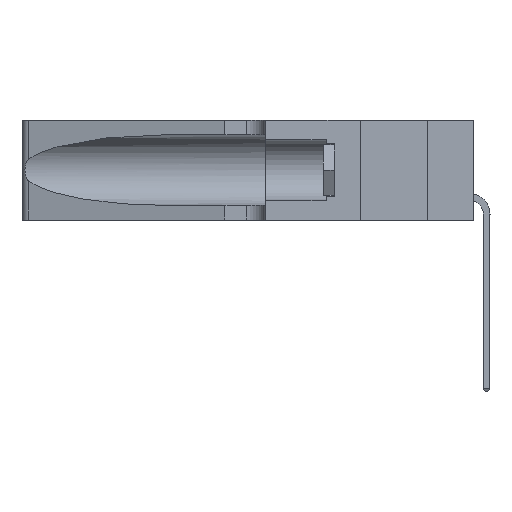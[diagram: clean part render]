
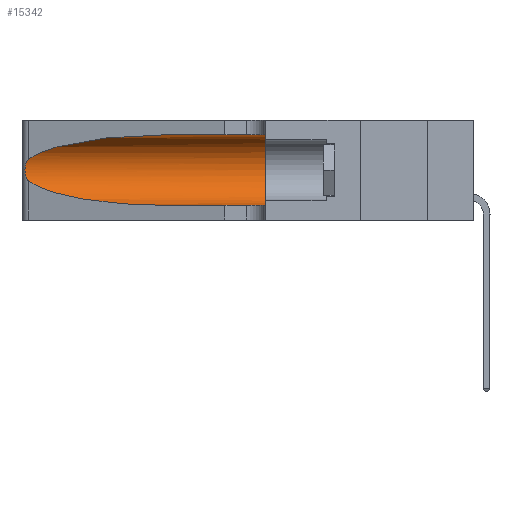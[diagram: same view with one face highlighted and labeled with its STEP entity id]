
A CAD part, left-side view. The second image highlights one B-rep face of the part: STEP entity #15342.
In plain terms, the highlighted cylindrical face has radius 3.308 mm (diameter 6.617 mm), a partial arc.
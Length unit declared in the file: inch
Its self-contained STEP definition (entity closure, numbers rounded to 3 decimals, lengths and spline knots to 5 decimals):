
#10 = B_SPLINE_CURVE_WITH_KNOTS ( 'NONE', 3,
 ( #20231, #10800, #4668, #15788, #2941, #12462, #14384, #12871, #17435, #11341, #9580, #4878, #15926, #14451 ),
 .UNSPECIFIED., .F., .F.,
 ( 4, 2, 2, 2, 2, 2, 4 ),
 ( 0., 0.00027, 0.00053, 0.00107, 0.0016, 0.00187, 0.00214 ),
 .UNSPECIFIED. ) ;
#601 = ORIENTED_EDGE ( 'NONE', *, *, #5058, .T. ) ;
#1097 = AXIS2_PLACEMENT_3D ( 'NONE', #1220, #7774, #7566 ) ;
#1220 = CARTESIAN_POINT ( 'NONE',  ( 0.1305, 0.35, 0.185 ) ) ;
#1369 = VERTEX_POINT ( 'NONE', #12164 ) ;
#1884 = CARTESIAN_POINT ( 'NONE',  ( 0.18966, 0.96281, 0.31525 ) ) ;
#2132 = DIRECTION ( 'NONE',  ( 0., 0., -1. ) ) ;
#2319 = CARTESIAN_POINT ( 'NONE',  ( 0.25487, 1.22718, 0.22369 ) ) ;
#2742 = CARTESIAN_POINT ( 'NONE',  ( 0.1305, 1.61858, 0.31525 ) ) ;
#2941 = CARTESIAN_POINT ( 'NONE',  ( 0.25854, 1.2359, 0.20912 ) ) ;
#3533 = VERTEX_POINT ( 'NONE', #2319 ) ;
#4243 = EDGE_CURVE ( 'NONE', #11460, #1369, #17446, .T. ) ;
#4668 = CARTESIAN_POINT ( 'NONE',  ( 0.25639, 1.23184, 0.21858 ) ) ;
#4878 = CARTESIAN_POINT ( 'NONE',  ( 0.25639, 1.23186, 0.15144 ) ) ;
#5058 = EDGE_CURVE ( 'NONE', #3533, #11460, #10, .T. ) ;
#5115 = CARTESIAN_POINT ( 'NONE',  ( 0.1305, 0.35, 0.31525 ) ) ;
#5627 = VERTEX_POINT ( 'NONE', #8941 ) ;
#6149 = EDGE_CURVE ( 'NONE', #8811, #18917, #12539, .T. ) ;
#6348 = DIRECTION ( 'NONE',  ( 0., -1., 0. ) ) ;
#6776 = ORIENTED_EDGE ( 'NONE', *, *, #20018, .T. ) ;
#6941 = CARTESIAN_POINT ( 'NONE',  ( 0.18966, 0.96281, 0.05475 ) ) ;
#7340 = EDGE_CURVE ( 'NONE', #1369, #5627, #11021, .T. ) ;
#7566 = DIRECTION ( 'NONE',  ( 0., 0., 1. ) ) ;
#7774 = DIRECTION ( 'NONE',  ( 0., 1., 0. ) ) ;
#7825 = EDGE_CURVE ( 'NONE', #18917, #5627, #13225, .T. ) ;
#8082 =( BOUNDED_CURVE ( )  B_SPLINE_CURVE ( 3, ( #8178, #1884, #8108, #9747 ),
 .UNSPECIFIED., .F., .F. ) 
 B_SPLINE_CURVE_WITH_KNOTS ( ( 4, 4 ),
 ( 1.5708, 2.84003 ),
 .UNSPECIFIED. ) 
 CURVE ( )  GEOMETRIC_REPRESENTATION_ITEM ( )  RATIONAL_B_SPLINE_CURVE ( ( 1., 0.87, 0.87, 1. ) ) 
 REPRESENTATION_ITEM ( '' )  );
#8108 = CARTESIAN_POINT ( 'NONE',  ( 0.2373, 1.15595, 0.28018 ) ) ;
#8178 = CARTESIAN_POINT ( 'NONE',  ( 0.1305, 0.72297, 0.31525 ) ) ;
#8194 = CARTESIAN_POINT ( 'NONE',  ( 0.1305, 0.72297, 0.31525 ) ) ;
#8485 = ORIENTED_EDGE ( 'NONE', *, *, #7825, .F. ) ;
#8613 = CARTESIAN_POINT ( 'NONE',  ( 0.1305, 1.61858, 0.185 ) ) ;
#8811 = VERTEX_POINT ( 'NONE', #8194 ) ;
#8941 = CARTESIAN_POINT ( 'NONE',  ( 0.1305, 0.35, 0.05475 ) ) ;
#9384 = CARTESIAN_POINT ( 'NONE',  ( 0.2373, 1.15595, 0.08982 ) ) ;
#9580 = CARTESIAN_POINT ( 'NONE',  ( 0.25789, 1.23486, 0.15765 ) ) ;
#9747 = CARTESIAN_POINT ( 'NONE',  ( 0.25487, 1.22718, 0.22369 ) ) ;
#10800 = CARTESIAN_POINT ( 'NONE',  ( 0.25555, 1.22994, 0.2215 ) ) ;
#11021 = LINE ( 'NONE', #15819, #19888 ) ;
#11341 = CARTESIAN_POINT ( 'NONE',  ( 0.25856, 1.23593, 0.16098 ) ) ;
#11460 = VERTEX_POINT ( 'NONE', #17697 ) ;
#11747 = DIRECTION ( 'NONE',  ( 0., -1., 0. ) ) ;
#11995 = ORIENTED_EDGE ( 'NONE', *, *, #4243, .T. ) ;
#12164 = CARTESIAN_POINT ( 'NONE',  ( 0.1305, 0.72297, 0.05475 ) ) ;
#12462 = CARTESIAN_POINT ( 'NONE',  ( 0.26018, 1.23835, 0.19895 ) ) ;
#12469 = CARTESIAN_POINT ( 'NONE',  ( 0.25487, 1.22718, 0.14631 ) ) ;
#12539 = LINE ( 'NONE', #2742, #17978 ) ;
#12781 = EDGE_LOOP ( 'NONE', ( #6776, #601, #11995, #20378, #8485, #14394 ) ) ;
#12871 = CARTESIAN_POINT ( 'NONE',  ( 0.26075, 1.23896, 0.178 ) ) ;
#12925 = CYLINDRICAL_SURFACE ( 'NONE', #15602, 0.13025 ) ;
#13176 = FACE_OUTER_BOUND ( 'NONE', #12781, .T. ) ;
#13225 = CIRCLE ( 'NONE', #1097, 0.13025 ) ;
#14384 = CARTESIAN_POINT ( 'NONE',  ( 0.26075, 1.23896, 0.19203 ) ) ;
#14394 = ORIENTED_EDGE ( 'NONE', *, *, #6149, .F. ) ;
#14451 = CARTESIAN_POINT ( 'NONE',  ( 0.25487, 1.22718, 0.14631 ) ) ;
#15342 = ADVANCED_FACE ( 'NONE', ( #13176 ), #12925, .F. ) ;
#15512 = DIRECTION ( 'NONE',  ( 0., -1., 0. ) ) ;
#15602 = AXIS2_PLACEMENT_3D ( 'NONE', #8613, #11747, #2132 ) ;
#15788 = CARTESIAN_POINT ( 'NONE',  ( 0.25787, 1.23484, 0.2124 ) ) ;
#15819 = CARTESIAN_POINT ( 'NONE',  ( 0.1305, 1.61858, 0.05475 ) ) ;
#15926 = CARTESIAN_POINT ( 'NONE',  ( 0.25555, 1.22993, 0.14849 ) ) ;
#16460 = CARTESIAN_POINT ( 'NONE',  ( 0.1305, 0.72297, 0.05475 ) ) ;
#17435 = CARTESIAN_POINT ( 'NONE',  ( 0.26017, 1.23833, 0.17102 ) ) ;
#17446 =( BOUNDED_CURVE ( )  B_SPLINE_CURVE ( 3, ( #12469, #9384, #6941, #16460 ),
 .UNSPECIFIED., .F., .F. ) 
 B_SPLINE_CURVE_WITH_KNOTS ( ( 4, 4 ),
 ( 3.44316, 4.71239 ),
 .UNSPECIFIED. ) 
 CURVE ( )  GEOMETRIC_REPRESENTATION_ITEM ( )  RATIONAL_B_SPLINE_CURVE ( ( 1., 0.87, 0.87, 1. ) ) 
 REPRESENTATION_ITEM ( '' )  );
#17697 = CARTESIAN_POINT ( 'NONE',  ( 0.25487, 1.22718, 0.14631 ) ) ;
#17978 = VECTOR ( 'NONE', #15512, 39.37008 ) ;
#18917 = VERTEX_POINT ( 'NONE', #5115 ) ;
#19888 = VECTOR ( 'NONE', #6348, 39.37008 ) ;
#20018 = EDGE_CURVE ( 'NONE', #8811, #3533, #8082, .T. ) ;
#20231 = CARTESIAN_POINT ( 'NONE',  ( 0.25487, 1.22718, 0.22369 ) ) ;
#20378 = ORIENTED_EDGE ( 'NONE', *, *, #7340, .T. ) ;
